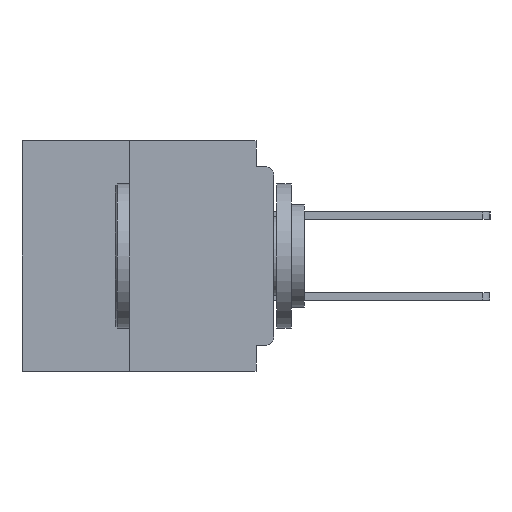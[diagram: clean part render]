
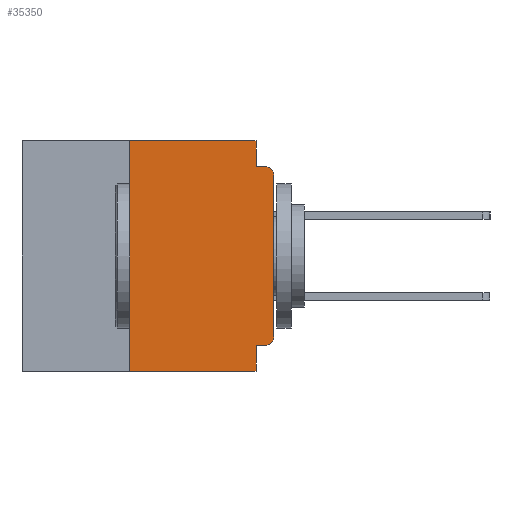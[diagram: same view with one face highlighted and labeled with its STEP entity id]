
A CAD part, left-side view. The second image highlights one B-rep face of the part: STEP entity #35350.
In plain terms, the highlighted planar face has unit normal (-1, 0, 0).
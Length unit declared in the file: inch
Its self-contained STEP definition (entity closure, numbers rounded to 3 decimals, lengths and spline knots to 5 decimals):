
#269 = CARTESIAN_POINT ( 'NONE',  ( 0., 0.031, -0.4 ) ) ;
#453 = VERTEX_POINT ( 'NONE', #45051 ) ;
#796 = DIRECTION ( 'NONE',  ( 0., 0., -1. ) ) ;
#1671 = EDGE_CURVE ( 'NONE', #9457, #453, #30491, .T. ) ;
#3178 = LINE ( 'NONE', #22867, #43377 ) ;
#3799 = EDGE_CURVE ( 'NONE', #7395, #37029, #43461, .T. ) ;
#4620 = CARTESIAN_POINT ( 'NONE',  ( 0., 0.015, -0.34 ) ) ;
#4652 = CARTESIAN_POINT ( 'NONE',  ( 0., 0.031, -0.045 ) ) ;
#5329 = CARTESIAN_POINT ( 'NONE',  ( 0., 0.25, -0.4 ) ) ;
#5401 = EDGE_CURVE ( 'NONE', #453, #46555, #3178, .T. ) ;
#6468 = CARTESIAN_POINT ( 'NONE',  ( 0., 0., -0.045 ) ) ;
#6580 = AXIS2_PLACEMENT_3D ( 'NONE', #4620, #30307, #8374 ) ;
#7395 = VERTEX_POINT ( 'NONE', #16641 ) ;
#7983 = VERTEX_POINT ( 'NONE', #10517 ) ;
#8374 = DIRECTION ( 'NONE',  ( 0., 0., -1. ) ) ;
#9104 = DIRECTION ( 'NONE',  ( -1., 0., 0. ) ) ;
#9457 = VERTEX_POINT ( 'NONE', #15838 ) ;
#9820 = VECTOR ( 'NONE', #32134, 39.37008 ) ;
#10517 = CARTESIAN_POINT ( 'NONE',  ( 0., 0.015, -0.045 ) ) ;
#10529 = VERTEX_POINT ( 'NONE', #33034 ) ;
#11006 = ORIENTED_EDGE ( 'NONE', *, *, #27565, .F. ) ;
#11553 = EDGE_CURVE ( 'NONE', #37029, #10529, #35955, .T. ) ;
#11660 = CARTESIAN_POINT ( 'NONE',  ( 0., 0., 0. ) ) ;
#11721 = VERTEX_POINT ( 'NONE', #41716 ) ;
#12034 = VECTOR ( 'NONE', #30051, 39.37008 ) ;
#12778 = ORIENTED_EDGE ( 'NONE', *, *, #15767, .T. ) ;
#13341 = VECTOR ( 'NONE', #37356, 39.37008 ) ;
#14263 = VECTOR ( 'NONE', #30347, 39.37008 ) ;
#15066 = ORIENTED_EDGE ( 'NONE', *, *, #3799, .F. ) ;
#15700 = AXIS2_PLACEMENT_3D ( 'NONE', #31043, #9104, #34701 ) ;
#15767 = EDGE_CURVE ( 'NONE', #11721, #10529, #33662, .T. ) ;
#15838 = CARTESIAN_POINT ( 'NONE',  ( 0., 0.25, 0. ) ) ;
#16608 = CARTESIAN_POINT ( 'NONE',  ( 0., 0.437, 0. ) ) ;
#16641 = CARTESIAN_POINT ( 'NONE',  ( 0., 0.015, -0.355 ) ) ;
#17608 = VECTOR ( 'NONE', #26035, 39.37008 ) ;
#17637 = CARTESIAN_POINT ( 'NONE',  ( 0., 0., -0.34 ) ) ;
#17830 = VECTOR ( 'NONE', #42053, 39.37008 ) ;
#18003 = EDGE_LOOP ( 'NONE', ( #33346, #24197, #11006, #23034, #42537, #26499, #12778, #32267, #15066, #44250 ) ) ;
#20105 = LINE ( 'NONE', #5329, #17830 ) ;
#20241 = CARTESIAN_POINT ( 'NONE',  ( 0., 0.031, -0.355 ) ) ;
#20254 = DIRECTION ( 'NONE',  ( 1., 0., 0. ) ) ;
#21549 = EDGE_CURVE ( 'NONE', #37512, #7983, #26854, .T. ) ;
#21598 = DIRECTION ( 'NONE',  ( 0., -1., 0. ) ) ;
#22867 = CARTESIAN_POINT ( 'NONE',  ( 0., 0.031, 0. ) ) ;
#23034 = ORIENTED_EDGE ( 'NONE', *, *, #5401, .F. ) ;
#24197 = ORIENTED_EDGE ( 'NONE', *, *, #21549, .T. ) ;
#25321 = AXIS2_PLACEMENT_3D ( 'NONE', #16608, #20254, #45895 ) ;
#26035 = DIRECTION ( 'NONE',  ( 0., 0., -1. ) ) ;
#26499 = ORIENTED_EDGE ( 'NONE', *, *, #27350, .F. ) ;
#26638 = CARTESIAN_POINT ( 'NONE',  ( 0., 0., -0.06 ) ) ;
#26854 = CIRCLE ( 'NONE', #15700, 0.015 ) ;
#27350 = EDGE_CURVE ( 'NONE', #11721, #9457, #20105, .T. ) ;
#27565 = EDGE_CURVE ( 'NONE', #46555, #7983, #40162, .T. ) ;
#30051 = DIRECTION ( 'NONE',  ( 0., 0., 1. ) ) ;
#30307 = DIRECTION ( 'NONE',  ( -1., 0., 0. ) ) ;
#30320 = FACE_OUTER_BOUND ( 'NONE', #18003, .T. ) ;
#30347 = DIRECTION ( 'NONE',  ( 0., 1., 0. ) ) ;
#30491 = LINE ( 'NONE', #39388, #13341 ) ;
#31043 = CARTESIAN_POINT ( 'NONE',  ( 0., 0.015, -0.06 ) ) ;
#31783 = CIRCLE ( 'NONE', #6580, 0.015 ) ;
#32134 = DIRECTION ( 'NONE',  ( 0., -1., 0. ) ) ;
#32267 = ORIENTED_EDGE ( 'NONE', *, *, #11553, .F. ) ;
#32516 = CARTESIAN_POINT ( 'NONE',  ( 0., 0.437, -0.4 ) ) ;
#32545 = VECTOR ( 'NONE', #21598, 39.37008 ) ;
#33034 = CARTESIAN_POINT ( 'NONE',  ( 0., 0.031, -0.4 ) ) ;
#33346 = ORIENTED_EDGE ( 'NONE', *, *, #41983, .T. ) ;
#33662 = LINE ( 'NONE', #32516, #32545 ) ;
#34018 = CARTESIAN_POINT ( 'NONE',  ( 0., 0., -0.355 ) ) ;
#34701 = DIRECTION ( 'NONE',  ( 0., 0., -1. ) ) ;
#35350 = ADVANCED_FACE ( 'NONE', ( #30320 ), #38513, .F. ) ;
#35955 = LINE ( 'NONE', #269, #17608 ) ;
#37029 = VERTEX_POINT ( 'NONE', #20241 ) ;
#37356 = DIRECTION ( 'NONE',  ( 0., -1., 0. ) ) ;
#37512 = VERTEX_POINT ( 'NONE', #26638 ) ;
#38513 = PLANE ( 'NONE',  #25321 ) ;
#39388 = CARTESIAN_POINT ( 'NONE',  ( 0., 0.437, 0. ) ) ;
#39677 = VERTEX_POINT ( 'NONE', #17637 ) ;
#40063 = LINE ( 'NONE', #11660, #12034 ) ;
#40162 = LINE ( 'NONE', #6468, #9820 ) ;
#41716 = CARTESIAN_POINT ( 'NONE',  ( 0., 0.25, -0.4 ) ) ;
#41983 = EDGE_CURVE ( 'NONE', #39677, #37512, #40063, .T. ) ;
#42053 = DIRECTION ( 'NONE',  ( 0., 0., 1. ) ) ;
#42537 = ORIENTED_EDGE ( 'NONE', *, *, #1671, .F. ) ;
#43377 = VECTOR ( 'NONE', #796, 39.37008 ) ;
#43461 = LINE ( 'NONE', #34018, #14263 ) ;
#44250 = ORIENTED_EDGE ( 'NONE', *, *, #44775, .T. ) ;
#44775 = EDGE_CURVE ( 'NONE', #7395, #39677, #31783, .T. ) ;
#45051 = CARTESIAN_POINT ( 'NONE',  ( 0., 0.031, 0. ) ) ;
#45895 = DIRECTION ( 'NONE',  ( 0., 0., -1. ) ) ;
#46555 = VERTEX_POINT ( 'NONE', #4652 ) ;
